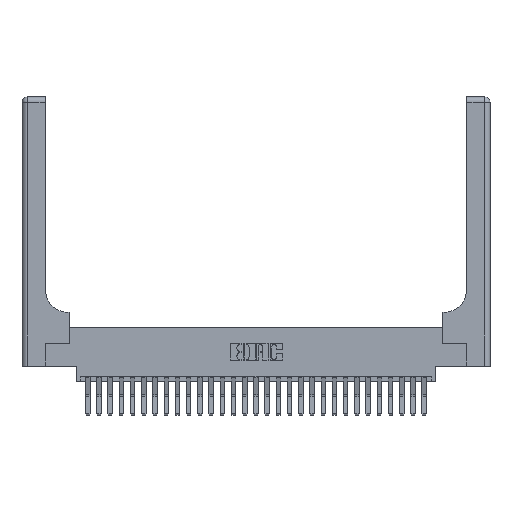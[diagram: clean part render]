
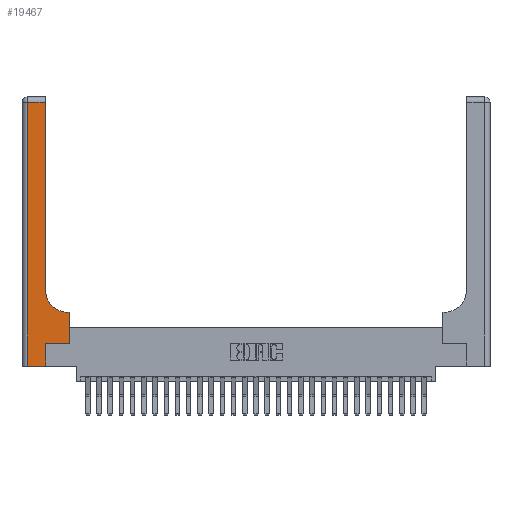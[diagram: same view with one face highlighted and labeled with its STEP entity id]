
A CAD part, top view. The second image highlights one B-rep face of the part: STEP entity #19467.
In plain terms, the highlighted planar face has unit normal (0, 0, 1).
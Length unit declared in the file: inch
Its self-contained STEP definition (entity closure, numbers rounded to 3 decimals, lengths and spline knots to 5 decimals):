
#887 = CARTESIAN_POINT ( 'NONE',  ( 0.265, 0.25, 0.37 ) ) ;
#970 = ORIENTED_EDGE ( 'NONE', *, *, #3462, .T. ) ;
#1016 = EDGE_CURVE ( 'NONE', #4722, #14652, #22348, .T. ) ;
#1426 = LINE ( 'NONE', #16737, #11516 ) ;
#1834 = CARTESIAN_POINT ( 'NONE',  ( 0.51, 0.6, 0.37 ) ) ;
#1936 = CARTESIAN_POINT ( 'NONE',  ( 0.06, 0., 0.37 ) ) ;
#2218 = CARTESIAN_POINT ( 'NONE',  ( 0.528, 0.25, 0.37 ) ) ;
#2594 = AXIS2_PLACEMENT_3D ( 'NONE', #24902, #7348, #14024 ) ;
#3462 = EDGE_CURVE ( 'NONE', #19914, #18280, #17338, .T. ) ;
#3728 = CARTESIAN_POINT ( 'NONE',  ( 0.26, 3., 0.37 ) ) ;
#3744 = ORIENTED_EDGE ( 'NONE', *, *, #18795, .T. ) ;
#3779 = ORIENTED_EDGE ( 'NONE', *, *, #4834, .T. ) ;
#3851 = ORIENTED_EDGE ( 'NONE', *, *, #22422, .T. ) ;
#4526 = VECTOR ( 'NONE', #26404, 39.37008 ) ;
#4722 = VERTEX_POINT ( 'NONE', #11491 ) ;
#4834 = EDGE_CURVE ( 'NONE', #8241, #4722, #24755, .T. ) ;
#4957 = AXIS2_PLACEMENT_3D ( 'NONE', #16787, #23476, #6341 ) ;
#5329 = VERTEX_POINT ( 'NONE', #5332 ) ;
#5332 = CARTESIAN_POINT ( 'NONE',  ( 0.528, 0.6, 0.37 ) ) ;
#5401 = CIRCLE ( 'NONE', #4957, 0.25 ) ;
#6285 = ORIENTED_EDGE ( 'NONE', *, *, #8748, .T. ) ;
#6297 = VECTOR ( 'NONE', #26141, 39.37008 ) ;
#6341 = DIRECTION ( 'NONE',  ( 1., 0., 0. ) ) ;
#6523 = EDGE_LOOP ( 'NONE', ( #6285, #970, #3744, #3779, #8033, #3851, #10051, #22014, #22111 ) ) ;
#6848 = VECTOR ( 'NONE', #20818, 39.37008 ) ;
#7348 = DIRECTION ( 'NONE',  ( 0., 0., -1. ) ) ;
#8033 = ORIENTED_EDGE ( 'NONE', *, *, #1016, .T. ) ;
#8241 = VERTEX_POINT ( 'NONE', #1936 ) ;
#8748 = EDGE_CURVE ( 'NONE', #27343, #19914, #16275, .T. ) ;
#9706 = VERTEX_POINT ( 'NONE', #1834 ) ;
#9937 = DIRECTION ( 'NONE',  ( -1., 0., 0. ) ) ;
#10051 = ORIENTED_EDGE ( 'NONE', *, *, #22093, .T. ) ;
#10220 = CARTESIAN_POINT ( 'NONE',  ( 0., 0., 0.37 ) ) ;
#10878 = DIRECTION ( 'NONE',  ( 0., 1., 0. ) ) ;
#11491 = CARTESIAN_POINT ( 'NONE',  ( 0.265, 0., 0.37 ) ) ;
#11516 = VECTOR ( 'NONE', #9937, 39.37008 ) ;
#12068 = PLANE ( 'NONE',  #2594 ) ;
#12193 = CARTESIAN_POINT ( 'NONE',  ( 0.06, 3., 0.37 ) ) ;
#13163 = LINE ( 'NONE', #887, #18825 ) ;
#14024 = DIRECTION ( 'NONE',  ( -1., 0., 0. ) ) ;
#14651 = VECTOR ( 'NONE', #18477, 39.37008 ) ;
#14652 = VERTEX_POINT ( 'NONE', #19020 ) ;
#16275 = LINE ( 'NONE', #3728, #16907 ) ;
#16737 = CARTESIAN_POINT ( 'NONE',  ( 0.26, 0.6, 0.37 ) ) ;
#16787 = CARTESIAN_POINT ( 'NONE',  ( 0.51, 0.85, 0.37 ) ) ;
#16907 = VECTOR ( 'NONE', #22564, 39.37008 ) ;
#17338 = LINE ( 'NONE', #19435, #6297 ) ;
#17845 = CARTESIAN_POINT ( 'NONE',  ( 0.06, 2.94, 0.37 ) ) ;
#17921 = DIRECTION ( 'NONE',  ( 1., 0., 0. ) ) ;
#18010 = EDGE_CURVE ( 'NONE', #5329, #9706, #1426, .T. ) ;
#18280 = VERTEX_POINT ( 'NONE', #17845 ) ;
#18477 = DIRECTION ( 'NONE',  ( 0., -1., 0. ) ) ;
#18741 = LINE ( 'NONE', #12193, #14651 ) ;
#18779 = VERTEX_POINT ( 'NONE', #22804 ) ;
#18795 = EDGE_CURVE ( 'NONE', #18280, #8241, #18741, .T. ) ;
#18825 = VECTOR ( 'NONE', #17921, 39.37008 ) ;
#19020 = CARTESIAN_POINT ( 'NONE',  ( 0.265, 0.25, 0.37 ) ) ;
#19435 = CARTESIAN_POINT ( 'NONE',  ( 0., 2.94, 0.37 ) ) ;
#19467 = ADVANCED_FACE ( 'NONE', ( #26725 ), #12068, .F. ) ;
#19914 = VERTEX_POINT ( 'NONE', #22503 ) ;
#20818 = DIRECTION ( 'NONE',  ( 1., 0., 0. ) ) ;
#21311 = LINE ( 'NONE', #2218, #25999 ) ;
#22014 = ORIENTED_EDGE ( 'NONE', *, *, #18010, .T. ) ;
#22093 = EDGE_CURVE ( 'NONE', #18779, #5329, #21311, .T. ) ;
#22111 = ORIENTED_EDGE ( 'NONE', *, *, #23444, .T. ) ;
#22348 = LINE ( 'NONE', #22489, #4526 ) ;
#22422 = EDGE_CURVE ( 'NONE', #14652, #18779, #13163, .T. ) ;
#22423 = CARTESIAN_POINT ( 'NONE',  ( 0.26, 0.85, 0.37 ) ) ;
#22489 = CARTESIAN_POINT ( 'NONE',  ( 0.265, 0., 0.37 ) ) ;
#22503 = CARTESIAN_POINT ( 'NONE',  ( 0.26, 2.94, 0.37 ) ) ;
#22564 = DIRECTION ( 'NONE',  ( 0., 1., 0. ) ) ;
#22804 = CARTESIAN_POINT ( 'NONE',  ( 0.528, 0.25, 0.37 ) ) ;
#23444 = EDGE_CURVE ( 'NONE', #9706, #27343, #5401, .T. ) ;
#23476 = DIRECTION ( 'NONE',  ( 0., 0., -1. ) ) ;
#24755 = LINE ( 'NONE', #10220, #6848 ) ;
#24902 = CARTESIAN_POINT ( 'NONE',  ( 0., 3., 0.37 ) ) ;
#25999 = VECTOR ( 'NONE', #10878, 39.37008 ) ;
#26141 = DIRECTION ( 'NONE',  ( -1., 0., 0. ) ) ;
#26404 = DIRECTION ( 'NONE',  ( 0., 1., 0. ) ) ;
#26725 = FACE_OUTER_BOUND ( 'NONE', #6523, .T. ) ;
#27343 = VERTEX_POINT ( 'NONE', #22423 ) ;
